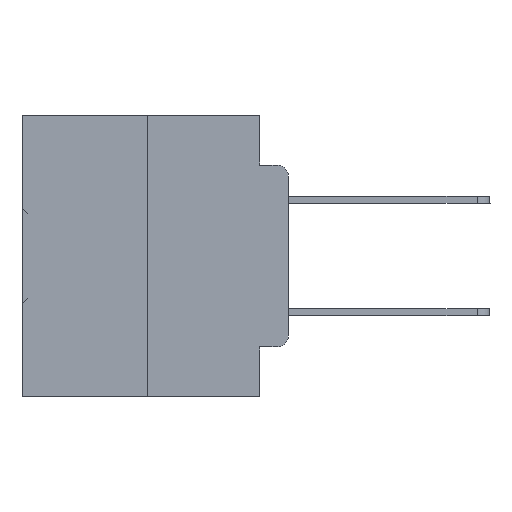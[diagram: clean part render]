
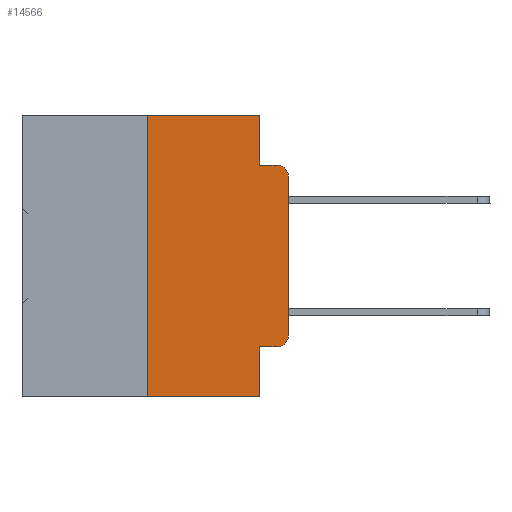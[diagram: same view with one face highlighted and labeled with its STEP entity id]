
A CAD part, left-side view. The second image highlights one B-rep face of the part: STEP entity #14566.
In plain terms, the highlighted planar face has unit normal (-1, 0, 0).
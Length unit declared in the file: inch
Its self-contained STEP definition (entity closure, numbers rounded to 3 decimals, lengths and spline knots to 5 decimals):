
#445 = CARTESIAN_POINT ( 'NONE',  ( 0., 0.25, 0. ) ) ;
#677 = CARTESIAN_POINT ( 'NONE',  ( 0., 0.25, -0.5 ) ) ;
#1395 = DIRECTION ( 'NONE',  ( 0., 0., -1. ) ) ;
#1463 = CARTESIAN_POINT ( 'NONE',  ( 0., 0.051, 0. ) ) ;
#1650 = EDGE_CURVE ( 'NONE', #28970, #17709, #26184, .T. ) ;
#2389 = LINE ( 'NONE', #28685, #29196 ) ;
#2990 = CARTESIAN_POINT ( 'NONE',  ( 0., 0.473, 0. ) ) ;
#3714 = EDGE_CURVE ( 'NONE', #28970, #7738, #2389, .T. ) ;
#4129 = VERTEX_POINT ( 'NONE', #36660 ) ;
#4173 = AXIS2_PLACEMENT_3D ( 'NONE', #7137, #15499, #1395 ) ;
#4490 = VERTEX_POINT ( 'NONE', #26986 ) ;
#4695 = DIRECTION ( 'NONE',  ( 0., 0., -1. ) ) ;
#4882 = VECTOR ( 'NONE', #25012, 39.37008 ) ;
#5608 = LINE ( 'NONE', #25590, #21196 ) ;
#5629 = EDGE_CURVE ( 'NONE', #28245, #16481, #14334, .T. ) ;
#6500 = VECTOR ( 'NONE', #4695, 39.37008 ) ;
#6736 = ORIENTED_EDGE ( 'NONE', *, *, #5629, .T. ) ;
#7102 = LINE ( 'NONE', #10080, #14279 ) ;
#7137 = CARTESIAN_POINT ( 'NONE',  ( 0., 0.02, -0.3915 ) ) ;
#7738 = VERTEX_POINT ( 'NONE', #10751 ) ;
#8298 = ORIENTED_EDGE ( 'NONE', *, *, #3714, .T. ) ;
#8487 = CARTESIAN_POINT ( 'NONE',  ( 0., 0.051, -0.4115 ) ) ;
#9562 = EDGE_CURVE ( 'NONE', #10699, #28245, #5608, .T. ) ;
#10019 = DIRECTION ( 'NONE',  ( -1., 0., 0. ) ) ;
#10080 = CARTESIAN_POINT ( 'NONE',  ( 0., 0.051, -0.0885 ) ) ;
#10656 = LINE ( 'NONE', #1463, #6500 ) ;
#10699 = VERTEX_POINT ( 'NONE', #22164 ) ;
#10751 = CARTESIAN_POINT ( 'NONE',  ( 0., 0.051, -0.5 ) ) ;
#10768 = ORIENTED_EDGE ( 'NONE', *, *, #26279, .F. ) ;
#10951 = CARTESIAN_POINT ( 'NONE',  ( 0., 0.473, 0. ) ) ;
#11171 = ORIENTED_EDGE ( 'NONE', *, *, #19391, .F. ) ;
#11639 = ORIENTED_EDGE ( 'NONE', *, *, #21766, .T. ) ;
#12376 = FACE_OUTER_BOUND ( 'NONE', #18911, .T. ) ;
#13011 = AXIS2_PLACEMENT_3D ( 'NONE', #21621, #10019, #13028 ) ;
#13028 = DIRECTION ( 'NONE',  ( 0., 0., -1. ) ) ;
#14279 = VECTOR ( 'NONE', #27301, 39.37008 ) ;
#14334 = CIRCLE ( 'NONE', #13011, 0.02 ) ;
#14566 = ADVANCED_FACE ( 'NONE', ( #12376 ), #20091, .F. ) ;
#15499 = DIRECTION ( 'NONE',  ( -1., 0., 0. ) ) ;
#15590 = ORIENTED_EDGE ( 'NONE', *, *, #36314, .T. ) ;
#16481 = VERTEX_POINT ( 'NONE', #34374 ) ;
#17492 = DIRECTION ( 'NONE',  ( 0., 0., 1. ) ) ;
#17709 = VERTEX_POINT ( 'NONE', #25258 ) ;
#18087 = CIRCLE ( 'NONE', #4173, 0.02 ) ;
#18592 = VECTOR ( 'NONE', #17492, 39.37008 ) ;
#18911 = EDGE_LOOP ( 'NONE', ( #36363, #6736, #11171, #19213, #31758, #19368, #8298, #10768, #11639, #15590 ) ) ;
#19213 = ORIENTED_EDGE ( 'NONE', *, *, #33435, .F. ) ;
#19368 = ORIENTED_EDGE ( 'NONE', *, *, #1650, .F. ) ;
#19391 = EDGE_CURVE ( 'NONE', #4129, #16481, #7102, .T. ) ;
#19518 = EDGE_CURVE ( 'NONE', #17709, #4490, #22758, .T. ) ;
#19612 = DIRECTION ( 'NONE',  ( 0., 0., -1. ) ) ;
#20053 = VECTOR ( 'NONE', #22587, 39.37008 ) ;
#20091 = PLANE ( 'NONE',  #28782 ) ;
#21137 = VERTEX_POINT ( 'NONE', #33788 ) ;
#21196 = VECTOR ( 'NONE', #28386, 39.37008 ) ;
#21581 = DIRECTION ( 'NONE',  ( 0., 0., -1. ) ) ;
#21621 = CARTESIAN_POINT ( 'NONE',  ( 0., 0.02, -0.1085 ) ) ;
#21766 = EDGE_CURVE ( 'NONE', #29986, #21137, #24515, .T. ) ;
#22164 = CARTESIAN_POINT ( 'NONE',  ( 0., 0., -0.3915 ) ) ;
#22587 = DIRECTION ( 'NONE',  ( 0., -1., 0. ) ) ;
#22758 = LINE ( 'NONE', #10951, #4882 ) ;
#22761 = VECTOR ( 'NONE', #21581, 39.37008 ) ;
#23035 = DIRECTION ( 'NONE',  ( 0., -1., 0. ) ) ;
#24051 = LINE ( 'NONE', #33600, #22761 ) ;
#24515 = LINE ( 'NONE', #8487, #20053 ) ;
#25012 = DIRECTION ( 'NONE',  ( 0., -1., 0. ) ) ;
#25258 = CARTESIAN_POINT ( 'NONE',  ( 0., 0.25, 0. ) ) ;
#25590 = CARTESIAN_POINT ( 'NONE',  ( 0., 0., 0. ) ) ;
#26184 = LINE ( 'NONE', #445, #18592 ) ;
#26279 = EDGE_CURVE ( 'NONE', #29986, #7738, #10656, .T. ) ;
#26986 = CARTESIAN_POINT ( 'NONE',  ( 0., 0.051, 0. ) ) ;
#27301 = DIRECTION ( 'NONE',  ( 0., -1., 0. ) ) ;
#28245 = VERTEX_POINT ( 'NONE', #34942 ) ;
#28386 = DIRECTION ( 'NONE',  ( 0., 0., 1. ) ) ;
#28685 = CARTESIAN_POINT ( 'NONE',  ( 0., 0.473, -0.5 ) ) ;
#28782 = AXIS2_PLACEMENT_3D ( 'NONE', #2990, #36742, #19612 ) ;
#28970 = VERTEX_POINT ( 'NONE', #677 ) ;
#29196 = VECTOR ( 'NONE', #23035, 39.37008 ) ;
#29986 = VERTEX_POINT ( 'NONE', #34583 ) ;
#31758 = ORIENTED_EDGE ( 'NONE', *, *, #19518, .F. ) ;
#33435 = EDGE_CURVE ( 'NONE', #4490, #4129, #24051, .T. ) ;
#33600 = CARTESIAN_POINT ( 'NONE',  ( 0., 0.051, 0. ) ) ;
#33788 = CARTESIAN_POINT ( 'NONE',  ( 0., 0.02, -0.4115 ) ) ;
#34374 = CARTESIAN_POINT ( 'NONE',  ( 0., 0.02, -0.0885 ) ) ;
#34583 = CARTESIAN_POINT ( 'NONE',  ( 0., 0.051, -0.4115 ) ) ;
#34942 = CARTESIAN_POINT ( 'NONE',  ( 0., 0., -0.1085 ) ) ;
#36314 = EDGE_CURVE ( 'NONE', #21137, #10699, #18087, .T. ) ;
#36363 = ORIENTED_EDGE ( 'NONE', *, *, #9562, .T. ) ;
#36660 = CARTESIAN_POINT ( 'NONE',  ( 0., 0.051, -0.0885 ) ) ;
#36742 = DIRECTION ( 'NONE',  ( 1., 0., 0. ) ) ;
